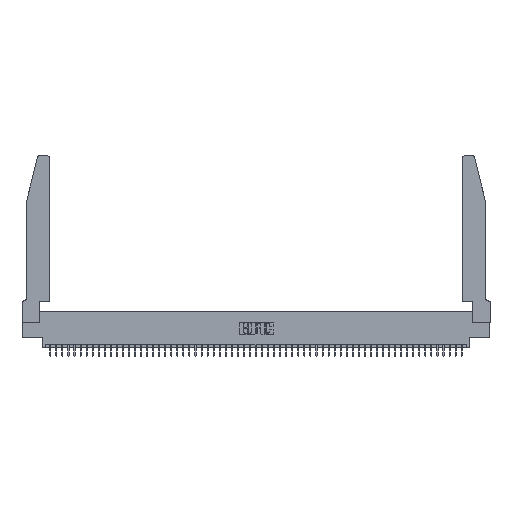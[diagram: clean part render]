
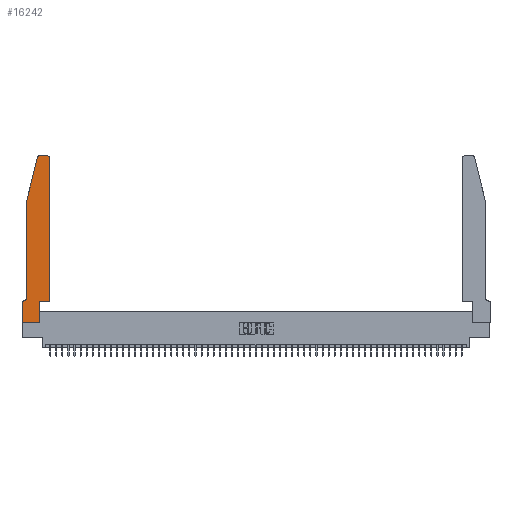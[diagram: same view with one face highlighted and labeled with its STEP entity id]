
A CAD part, top view. The second image highlights one B-rep face of the part: STEP entity #16242.
In plain terms, the highlighted planar face has unit normal (0, 0, 1).
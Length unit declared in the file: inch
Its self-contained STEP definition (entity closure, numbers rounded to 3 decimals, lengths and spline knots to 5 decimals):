
#390 = EDGE_LOOP ( 'NONE', ( #879, #7094, #37255, #22807, #22083, #35553, #32328, #21849, #30283, #35843, #38863, #47273 ) ) ;
#709 = VECTOR ( 'NONE', #7404, 39.37008 ) ;
#879 = ORIENTED_EDGE ( 'NONE', *, *, #8395, .T. ) ;
#1189 = AXIS2_PLACEMENT_3D ( 'NONE', #15500, #45544, #28400 ) ;
#1407 = VERTEX_POINT ( 'NONE', #22524 ) ;
#2209 = VERTEX_POINT ( 'NONE', #20749 ) ;
#2350 = CARTESIAN_POINT ( 'NONE',  ( 0.4505, 0.35, 0.37 ) ) ;
#2447 = CARTESIAN_POINT ( 'NONE',  ( 0.2605, 2.75, 0.37 ) ) ;
#2911 = LINE ( 'NONE', #2350, #709 ) ;
#3615 = LINE ( 'NONE', #12611, #17186 ) ;
#4477 = CARTESIAN_POINT ( 'NONE',  ( 0.0755, 2., 0.37 ) ) ;
#4855 = CIRCLE ( 'NONE', #17435, 0.07 ) ;
#5033 = LINE ( 'NONE', #47775, #24117 ) ;
#7094 = ORIENTED_EDGE ( 'NONE', *, *, #13415, .T. ) ;
#7108 = AXIS2_PLACEMENT_3D ( 'NONE', #44946, #19378, #10940 ) ;
#7404 = DIRECTION ( 'NONE',  ( 0., 1., 0. ) ) ;
#7949 = DIRECTION ( 'NONE',  ( 0., 0., -1. ) ) ;
#8395 = EDGE_CURVE ( 'NONE', #42282, #2209, #45741, .T. ) ;
#9100 = VERTEX_POINT ( 'NONE', #23605 ) ;
#9994 = AXIS2_PLACEMENT_3D ( 'NONE', #28601, #11204, #49692 ) ;
#10940 = DIRECTION ( 'NONE',  ( 1., 0., 0. ) ) ;
#11204 = DIRECTION ( 'NONE',  ( 0., 0., 1. ) ) ;
#11312 = DIRECTION ( 'NONE',  ( 1., 0., 0. ) ) ;
#12405 = CARTESIAN_POINT ( 'NONE',  ( 0., 0.35, 0.37 ) ) ;
#12611 = CARTESIAN_POINT ( 'NONE',  ( 0.0755, 2., 0.37 ) ) ;
#13415 = EDGE_CURVE ( 'NONE', #2209, #40271, #25379, .T. ) ;
#13469 = VECTOR ( 'NONE', #45961, 39.37008 ) ;
#14698 = VERTEX_POINT ( 'NONE', #37378 ) ;
#15452 = EDGE_CURVE ( 'NONE', #1407, #23736, #2911, .T. ) ;
#15500 = CARTESIAN_POINT ( 'NONE',  ( 0.4205, 2.72, 0.37 ) ) ;
#15934 = CARTESIAN_POINT ( 'NONE',  ( 0., 0., 0.37 ) ) ;
#16007 = DIRECTION ( 'NONE',  ( 0., -1., 0. ) ) ;
#16077 = EDGE_CURVE ( 'NONE', #36386, #40661, #5033, .T. ) ;
#16242 = ADVANCED_FACE ( 'NONE', ( #53907 ), #23599, .T. ) ;
#17186 = VECTOR ( 'NONE', #16007, 39.37008 ) ;
#17435 = AXIS2_PLACEMENT_3D ( 'NONE', #30669, #7949, #29860 ) ;
#17458 = DIRECTION ( 'NONE',  ( 0., 1., 0. ) ) ;
#17505 = VERTEX_POINT ( 'NONE', #36963 ) ;
#17716 = DIRECTION ( 'NONE',  ( -1., 0., 0. ) ) ;
#18392 = CARTESIAN_POINT ( 'NONE',  ( 0.4505, 2.72, 0.37 ) ) ;
#19378 = DIRECTION ( 'NONE',  ( 0., 0., 1. ) ) ;
#20749 = CARTESIAN_POINT ( 'NONE',  ( 0.284, 2.75, 0.37 ) ) ;
#20944 = VECTOR ( 'NONE', #47207, 39.37008 ) ;
#21113 = LINE ( 'NONE', #29255, #45157 ) ;
#21277 = EDGE_CURVE ( 'NONE', #14698, #9100, #21113, .T. ) ;
#21702 = VECTOR ( 'NONE', #25171, 39.37008 ) ;
#21849 = ORIENTED_EDGE ( 'NONE', *, *, #48617, .T. ) ;
#22083 = ORIENTED_EDGE ( 'NONE', *, *, #24070, .T. ) ;
#22524 = CARTESIAN_POINT ( 'NONE',  ( 0.4505, 0.35, 0.37 ) ) ;
#22807 = ORIENTED_EDGE ( 'NONE', *, *, #39122, .T. ) ;
#23106 = CARTESIAN_POINT ( 'NONE',  ( 0.25487, 2.72718, 0.37 ) ) ;
#23599 = PLANE ( 'NONE',  #7108 ) ;
#23605 = CARTESIAN_POINT ( 'NONE',  ( 0.2865, 0.35, 0.37 ) ) ;
#23736 = VERTEX_POINT ( 'NONE', #18392 ) ;
#24070 = EDGE_CURVE ( 'NONE', #17505, #36386, #4855, .T. ) ;
#24117 = VECTOR ( 'NONE', #17716, 39.37008 ) ;
#24266 = VERTEX_POINT ( 'NONE', #30946 ) ;
#24888 = LINE ( 'NONE', #15934, #21702 ) ;
#25171 = DIRECTION ( 'NONE',  ( 1., 0., 0. ) ) ;
#25379 = CIRCLE ( 'NONE', #9994, 0.03 ) ;
#28400 = DIRECTION ( 'NONE',  ( 1., 0., 0. ) ) ;
#28457 = CARTESIAN_POINT ( 'NONE',  ( 0.0055, 0.35, 0.37 ) ) ;
#28601 = CARTESIAN_POINT ( 'NONE',  ( 0.284, 2.72, 0.37 ) ) ;
#28797 = CARTESIAN_POINT ( 'NONE',  ( 0., 0., 0.37 ) ) ;
#29024 = VECTOR ( 'NONE', #49682, 39.37008 ) ;
#29255 = CARTESIAN_POINT ( 'NONE',  ( 0.2865, 0.35, 0.37 ) ) ;
#29497 = LINE ( 'NONE', #4477, #20944 ) ;
#29860 = DIRECTION ( 'NONE',  ( -1., 0., 0. ) ) ;
#30283 = ORIENTED_EDGE ( 'NONE', *, *, #21277, .T. ) ;
#30639 = VERTEX_POINT ( 'NONE', #50983 ) ;
#30669 = CARTESIAN_POINT ( 'NONE',  ( 0.0055, 0.42, 0.37 ) ) ;
#30946 = CARTESIAN_POINT ( 'NONE',  ( 0., 0., 0.37 ) ) ;
#32328 = ORIENTED_EDGE ( 'NONE', *, *, #46468, .T. ) ;
#35026 = EDGE_CURVE ( 'NONE', #9100, #1407, #41639, .T. ) ;
#35553 = ORIENTED_EDGE ( 'NONE', *, *, #16077, .T. ) ;
#35843 = ORIENTED_EDGE ( 'NONE', *, *, #35026, .T. ) ;
#36386 = VERTEX_POINT ( 'NONE', #28457 ) ;
#36963 = CARTESIAN_POINT ( 'NONE',  ( 0.0755, 0.42, 0.37 ) ) ;
#37255 = ORIENTED_EDGE ( 'NONE', *, *, #52347, .T. ) ;
#37378 = CARTESIAN_POINT ( 'NONE',  ( 0.2865, 0., 0.37 ) ) ;
#38863 = ORIENTED_EDGE ( 'NONE', *, *, #15452, .T. ) ;
#39122 = EDGE_CURVE ( 'NONE', #30639, #17505, #3615, .T. ) ;
#40271 = VERTEX_POINT ( 'NONE', #23106 ) ;
#40661 = VERTEX_POINT ( 'NONE', #12405 ) ;
#41639 = LINE ( 'NONE', #49810, #44779 ) ;
#42282 = VERTEX_POINT ( 'NONE', #52168 ) ;
#43361 = CIRCLE ( 'NONE', #1189, 0.03 ) ;
#44779 = VECTOR ( 'NONE', #11312, 39.37008 ) ;
#44946 = CARTESIAN_POINT ( 'NONE',  ( 0., 0.35, 0.37 ) ) ;
#45157 = VECTOR ( 'NONE', #17458, 39.37008 ) ;
#45544 = DIRECTION ( 'NONE',  ( 0., 0., 1. ) ) ;
#45741 = LINE ( 'NONE', #2447, #29024 ) ;
#45961 = DIRECTION ( 'NONE',  ( 0., -1., 0. ) ) ;
#46468 = EDGE_CURVE ( 'NONE', #40661, #24266, #50439, .T. ) ;
#47207 = DIRECTION ( 'NONE',  ( -0.239, -0.971, 0. ) ) ;
#47273 = ORIENTED_EDGE ( 'NONE', *, *, #52127, .T. ) ;
#47775 = CARTESIAN_POINT ( 'NONE',  ( 0.0755, 0.35, 0.37 ) ) ;
#48617 = EDGE_CURVE ( 'NONE', #24266, #14698, #24888, .T. ) ;
#49682 = DIRECTION ( 'NONE',  ( -1., 0., 0. ) ) ;
#49692 = DIRECTION ( 'NONE',  ( 1., 0., 0. ) ) ;
#49810 = CARTESIAN_POINT ( 'NONE',  ( 0.4505, 0.35, 0.37 ) ) ;
#50439 = LINE ( 'NONE', #28797, #13469 ) ;
#50983 = CARTESIAN_POINT ( 'NONE',  ( 0.0755, 2., 0.37 ) ) ;
#52127 = EDGE_CURVE ( 'NONE', #23736, #42282, #43361, .T. ) ;
#52168 = CARTESIAN_POINT ( 'NONE',  ( 0.4205, 2.75, 0.37 ) ) ;
#52347 = EDGE_CURVE ( 'NONE', #40271, #30639, #29497, .T. ) ;
#53907 = FACE_OUTER_BOUND ( 'NONE', #390, .T. ) ;
